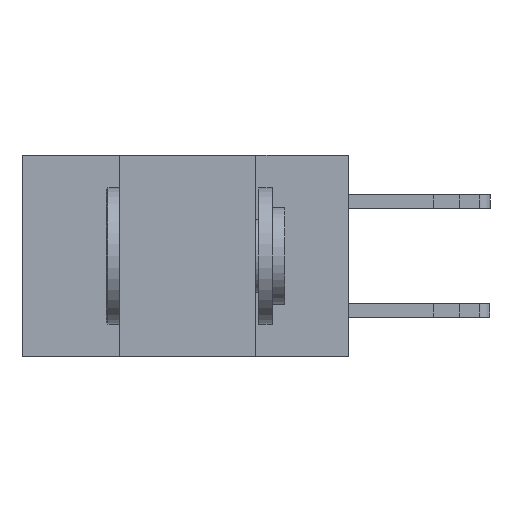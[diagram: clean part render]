
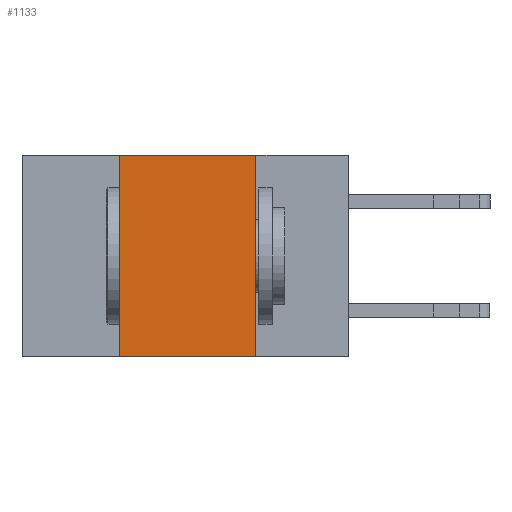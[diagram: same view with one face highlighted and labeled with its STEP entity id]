
A CAD part, left-side view. The second image highlights one B-rep face of the part: STEP entity #1133.
In plain terms, the highlighted planar face has unit normal (-1, 0, 0).
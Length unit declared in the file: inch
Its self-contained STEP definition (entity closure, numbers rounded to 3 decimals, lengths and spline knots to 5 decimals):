
#167 = VECTOR ( 'NONE', #2461, 39.37008 ) ;
#926 = DIRECTION ( 'NONE',  ( 0., 0., -1. ) ) ;
#1133 = ADVANCED_FACE ( 'NONE', ( #11248 ), #10453, .F. ) ;
#1260 = CARTESIAN_POINT ( 'NONE',  ( 0., 0.17, 0. ) ) ;
#1474 = LINE ( 'NONE', #15312, #8799 ) ;
#1633 = VERTEX_POINT ( 'NONE', #13831 ) ;
#2179 = DIRECTION ( 'NONE',  ( 0., 0., -1. ) ) ;
#2461 = DIRECTION ( 'NONE',  ( 0., -1., 0. ) ) ;
#2507 = CARTESIAN_POINT ( 'NONE',  ( 0., 0.42, -0.37 ) ) ;
#2562 = CARTESIAN_POINT ( 'NONE',  ( 0., 0.6, -0.37 ) ) ;
#4726 = EDGE_LOOP ( 'NONE', ( #7637, #16888, #14758, #17766 ) ) ;
#4896 = VERTEX_POINT ( 'NONE', #16382 ) ;
#5288 = EDGE_CURVE ( 'NONE', #17665, #1633, #9269, .T. ) ;
#6757 = VECTOR ( 'NONE', #926, 39.37008 ) ;
#6880 = EDGE_CURVE ( 'NONE', #12985, #17665, #1474, .T. ) ;
#7194 = EDGE_CURVE ( 'NONE', #1633, #4896, #17975, .T. ) ;
#7637 = ORIENTED_EDGE ( 'NONE', *, *, #7194, .F. ) ;
#8396 = EDGE_CURVE ( 'NONE', #12985, #4896, #11239, .T. ) ;
#8799 = VECTOR ( 'NONE', #14799, 39.37008 ) ;
#9269 = LINE ( 'NONE', #14448, #16742 ) ;
#10095 = DIRECTION ( 'NONE',  ( 1., 0., 0. ) ) ;
#10453 = PLANE ( 'NONE',  #10707 ) ;
#10707 = AXIS2_PLACEMENT_3D ( 'NONE', #13074, #10095, #2179 ) ;
#11239 = LINE ( 'NONE', #2562, #167 ) ;
#11248 = FACE_OUTER_BOUND ( 'NONE', #4726, .T. ) ;
#12985 = VERTEX_POINT ( 'NONE', #2507 ) ;
#13074 = CARTESIAN_POINT ( 'NONE',  ( 0., 0.6, 0. ) ) ;
#13831 = CARTESIAN_POINT ( 'NONE',  ( 0., 0.17, 0. ) ) ;
#14291 = CARTESIAN_POINT ( 'NONE',  ( 0., 0.42, 0. ) ) ;
#14305 = DIRECTION ( 'NONE',  ( 0., -1., 0. ) ) ;
#14448 = CARTESIAN_POINT ( 'NONE',  ( 0., 0.6, 0. ) ) ;
#14758 = ORIENTED_EDGE ( 'NONE', *, *, #6880, .F. ) ;
#14799 = DIRECTION ( 'NONE',  ( 0., 0., 1. ) ) ;
#15312 = CARTESIAN_POINT ( 'NONE',  ( 0., 0.42, 0. ) ) ;
#16382 = CARTESIAN_POINT ( 'NONE',  ( 0., 0.17, -0.37 ) ) ;
#16742 = VECTOR ( 'NONE', #14305, 39.37008 ) ;
#16888 = ORIENTED_EDGE ( 'NONE', *, *, #5288, .F. ) ;
#17665 = VERTEX_POINT ( 'NONE', #14291 ) ;
#17766 = ORIENTED_EDGE ( 'NONE', *, *, #8396, .T. ) ;
#17975 = LINE ( 'NONE', #1260, #6757 ) ;
